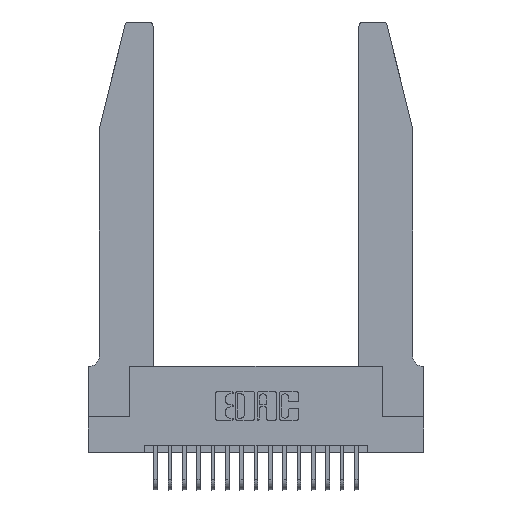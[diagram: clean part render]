
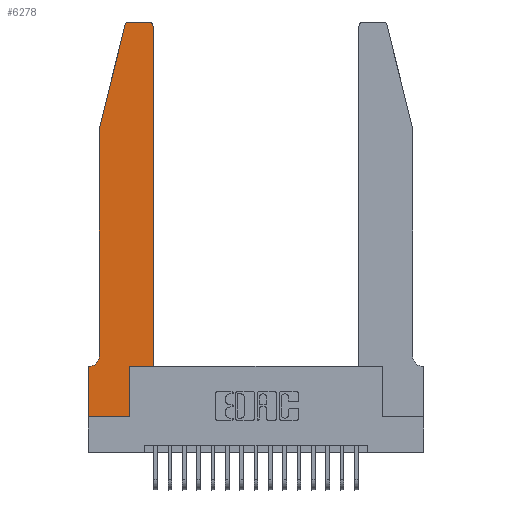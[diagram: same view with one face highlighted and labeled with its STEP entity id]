
A CAD part, top view. The second image highlights one B-rep face of the part: STEP entity #6278.
In plain terms, the highlighted planar face has unit normal (0, 0, 1).
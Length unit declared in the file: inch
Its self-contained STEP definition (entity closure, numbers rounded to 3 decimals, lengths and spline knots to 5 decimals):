
#196 = EDGE_CURVE ( 'NONE', #5476, #10379, #3943, .T. ) ;
#225 = LINE ( 'NONE', #21142, #19776 ) ;
#861 = EDGE_CURVE ( 'NONE', #18379, #17129, #20528, .T. ) ;
#1120 = ORIENTED_EDGE ( 'NONE', *, *, #16139, .T. ) ;
#1165 = LINE ( 'NONE', #16701, #12505 ) ;
#1246 = VERTEX_POINT ( 'NONE', #9808 ) ;
#2030 = ORIENTED_EDGE ( 'NONE', *, *, #13757, .T. ) ;
#2107 = DIRECTION ( 'NONE',  ( 0., 1., 0. ) ) ;
#2374 = CARTESIAN_POINT ( 'NONE',  ( 0., 0.35, 0.37 ) ) ;
#2393 = VERTEX_POINT ( 'NONE', #12395 ) ;
#2464 = CARTESIAN_POINT ( 'NONE',  ( 0.284, 2.72, 0.37 ) ) ;
#2488 = PLANE ( 'NONE',  #16326 ) ;
#2552 = CARTESIAN_POINT ( 'NONE',  ( 0., 0., 0.37 ) ) ;
#2642 = CARTESIAN_POINT ( 'NONE',  ( 0.2605, 2.75, 0.37 ) ) ;
#2782 = VERTEX_POINT ( 'NONE', #9444 ) ;
#3090 = CARTESIAN_POINT ( 'NONE',  ( 0., 0., 0.37 ) ) ;
#3463 = ORIENTED_EDGE ( 'NONE', *, *, #3814, .T. ) ;
#3523 = EDGE_CURVE ( 'NONE', #1246, #18379, #9158, .T. ) ;
#3769 = AXIS2_PLACEMENT_3D ( 'NONE', #13906, #17231, #17083 ) ;
#3772 = CARTESIAN_POINT ( 'NONE',  ( 0.4205, 2.75, 0.37 ) ) ;
#3814 = EDGE_CURVE ( 'NONE', #14398, #2393, #17615, .T. ) ;
#3943 = LINE ( 'NONE', #7231, #21325 ) ;
#3961 = ORIENTED_EDGE ( 'NONE', *, *, #15839, .T. ) ;
#4047 = ORIENTED_EDGE ( 'NONE', *, *, #16617, .T. ) ;
#4407 = ORIENTED_EDGE ( 'NONE', *, *, #3523, .T. ) ;
#5330 = CARTESIAN_POINT ( 'NONE',  ( 0.4505, 0.35, 0.37 ) ) ;
#5432 = VECTOR ( 'NONE', #15877, 39.37008 ) ;
#5476 = VERTEX_POINT ( 'NONE', #12619 ) ;
#5558 = CARTESIAN_POINT ( 'NONE',  ( 0.2865, 0.35, 0.37 ) ) ;
#6278 = ADVANCED_FACE ( 'NONE', ( #14037 ), #2488, .T. ) ;
#6608 = EDGE_CURVE ( 'NONE', #20157, #2782, #19617, .T. ) ;
#6634 = DIRECTION ( 'NONE',  ( 1., 0., 0. ) ) ;
#7091 = CARTESIAN_POINT ( 'NONE',  ( 0.0755, 0.35, 0.37 ) ) ;
#7176 = ORIENTED_EDGE ( 'NONE', *, *, #861, .T. ) ;
#7194 = ORIENTED_EDGE ( 'NONE', *, *, #12814, .T. ) ;
#7231 = CARTESIAN_POINT ( 'NONE',  ( 0.0755, 2., 0.37 ) ) ;
#7570 = CARTESIAN_POINT ( 'NONE',  ( 0., 0.35, 0.37 ) ) ;
#7626 = DIRECTION ( 'NONE',  ( 1., 0., 0. ) ) ;
#7842 = VECTOR ( 'NONE', #2107, 39.37008 ) ;
#8095 = AXIS2_PLACEMENT_3D ( 'NONE', #9372, #11285, #17955 ) ;
#8191 = CARTESIAN_POINT ( 'NONE',  ( 0.284, 2.75, 0.37 ) ) ;
#9019 = VECTOR ( 'NONE', #12816, 39.37008 ) ;
#9158 = CIRCLE ( 'NONE', #8095, 0.07 ) ;
#9176 = DIRECTION ( 'NONE',  ( -0.239, -0.971, 0. ) ) ;
#9214 = CARTESIAN_POINT ( 'NONE',  ( 0.0055, 0.35, 0.37 ) ) ;
#9354 = CARTESIAN_POINT ( 'NONE',  ( 0.0755, 2., 0.37 ) ) ;
#9372 = CARTESIAN_POINT ( 'NONE',  ( 0.0055, 0.42, 0.37 ) ) ;
#9444 = CARTESIAN_POINT ( 'NONE',  ( 0.2865, 0.35, 0.37 ) ) ;
#9598 = LINE ( 'NONE', #9354, #5432 ) ;
#9701 = VERTEX_POINT ( 'NONE', #3772 ) ;
#9808 = CARTESIAN_POINT ( 'NONE',  ( 0.0755, 0.42, 0.37 ) ) ;
#10147 = LINE ( 'NONE', #2642, #15194 ) ;
#10379 = VERTEX_POINT ( 'NONE', #11029 ) ;
#10453 = EDGE_CURVE ( 'NONE', #11161, #20157, #1165, .T. ) ;
#10734 = VECTOR ( 'NONE', #11114, 39.37008 ) ;
#10960 = CIRCLE ( 'NONE', #3769, 0.03 ) ;
#11029 = CARTESIAN_POINT ( 'NONE',  ( 0.0755, 2., 0.37 ) ) ;
#11114 = DIRECTION ( 'NONE',  ( -1., 0., 0. ) ) ;
#11161 = VERTEX_POINT ( 'NONE', #2552 ) ;
#11285 = DIRECTION ( 'NONE',  ( 0., 0., -1. ) ) ;
#11556 = DIRECTION ( 'NONE',  ( 0., -1., 0. ) ) ;
#11796 = AXIS2_PLACEMENT_3D ( 'NONE', #2464, #17092, #20296 ) ;
#11911 = LINE ( 'NONE', #3090, #14522 ) ;
#12257 = ORIENTED_EDGE ( 'NONE', *, *, #6608, .T. ) ;
#12395 = CARTESIAN_POINT ( 'NONE',  ( 0.4505, 2.72, 0.37 ) ) ;
#12505 = VECTOR ( 'NONE', #6634, 39.37008 ) ;
#12619 = CARTESIAN_POINT ( 'NONE',  ( 0.25487, 2.72718, 0.37 ) ) ;
#12723 = DIRECTION ( 'NONE',  ( 1., 0., 0. ) ) ;
#12814 = EDGE_CURVE ( 'NONE', #17129, #11161, #11911, .T. ) ;
#12816 = DIRECTION ( 'NONE',  ( 0., 1., 0. ) ) ;
#12976 = CARTESIAN_POINT ( 'NONE',  ( 0.2865, 0., 0.37 ) ) ;
#13109 = ORIENTED_EDGE ( 'NONE', *, *, #196, .T. ) ;
#13522 = VERTEX_POINT ( 'NONE', #8191 ) ;
#13757 = EDGE_CURVE ( 'NONE', #2782, #14398, #225, .T. ) ;
#13906 = CARTESIAN_POINT ( 'NONE',  ( 0.4205, 2.72, 0.37 ) ) ;
#14037 = FACE_OUTER_BOUND ( 'NONE', #21592, .T. ) ;
#14398 = VERTEX_POINT ( 'NONE', #5330 ) ;
#14522 = VECTOR ( 'NONE', #11556, 39.37008 ) ;
#14765 = EDGE_CURVE ( 'NONE', #13522, #5476, #16776, .T. ) ;
#15194 = VECTOR ( 'NONE', #21216, 39.37008 ) ;
#15839 = EDGE_CURVE ( 'NONE', #2393, #9701, #10960, .T. ) ;
#15877 = DIRECTION ( 'NONE',  ( 0., -1., 0. ) ) ;
#16139 = EDGE_CURVE ( 'NONE', #9701, #13522, #10147, .T. ) ;
#16326 = AXIS2_PLACEMENT_3D ( 'NONE', #7570, #21076, #12723 ) ;
#16617 = EDGE_CURVE ( 'NONE', #10379, #1246, #9598, .T. ) ;
#16701 = CARTESIAN_POINT ( 'NONE',  ( 0., 0., 0.37 ) ) ;
#16776 = CIRCLE ( 'NONE', #11796, 0.03 ) ;
#17083 = DIRECTION ( 'NONE',  ( 1., 0., 0. ) ) ;
#17092 = DIRECTION ( 'NONE',  ( 0., 0., 1. ) ) ;
#17129 = VERTEX_POINT ( 'NONE', #2374 ) ;
#17231 = DIRECTION ( 'NONE',  ( 0., 0., 1. ) ) ;
#17410 = ORIENTED_EDGE ( 'NONE', *, *, #14765, .T. ) ;
#17615 = LINE ( 'NONE', #20626, #7842 ) ;
#17955 = DIRECTION ( 'NONE',  ( -1., 0., 0. ) ) ;
#18379 = VERTEX_POINT ( 'NONE', #9214 ) ;
#19617 = LINE ( 'NONE', #5558, #9019 ) ;
#19776 = VECTOR ( 'NONE', #7626, 39.37008 ) ;
#20157 = VERTEX_POINT ( 'NONE', #12976 ) ;
#20296 = DIRECTION ( 'NONE',  ( 1., 0., 0. ) ) ;
#20528 = LINE ( 'NONE', #7091, #10734 ) ;
#20626 = CARTESIAN_POINT ( 'NONE',  ( 0.4505, 0.35, 0.37 ) ) ;
#20847 = ORIENTED_EDGE ( 'NONE', *, *, #10453, .T. ) ;
#21076 = DIRECTION ( 'NONE',  ( 0., 0., 1. ) ) ;
#21142 = CARTESIAN_POINT ( 'NONE',  ( 0.4505, 0.35, 0.37 ) ) ;
#21216 = DIRECTION ( 'NONE',  ( -1., 0., 0. ) ) ;
#21325 = VECTOR ( 'NONE', #9176, 39.37008 ) ;
#21592 = EDGE_LOOP ( 'NONE', ( #1120, #17410, #13109, #4047, #4407, #7176, #7194, #20847, #12257, #2030, #3463, #3961 ) ) ;
